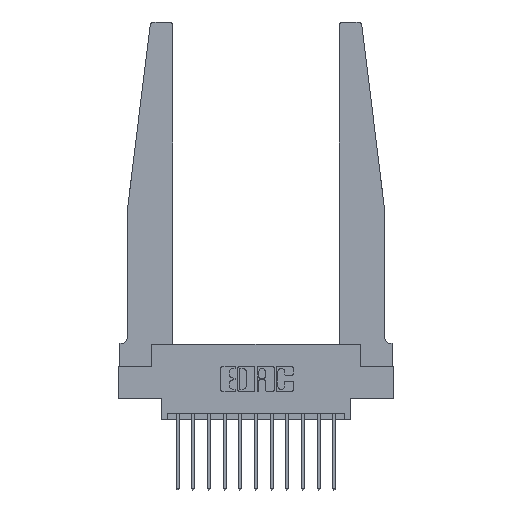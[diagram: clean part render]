
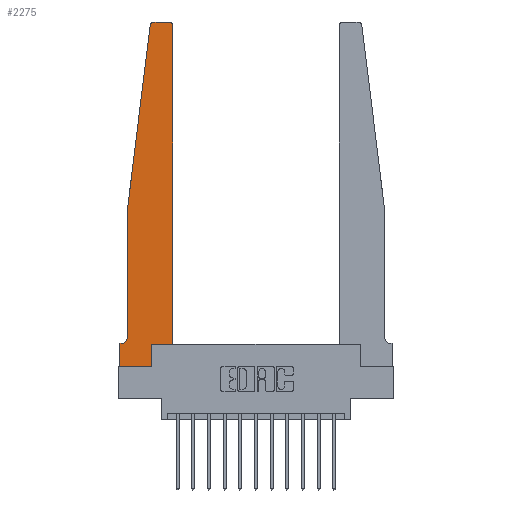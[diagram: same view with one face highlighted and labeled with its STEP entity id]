
A CAD part, top view. The second image highlights one B-rep face of the part: STEP entity #2275.
In plain terms, the highlighted planar face has unit normal (0, 0, 1).
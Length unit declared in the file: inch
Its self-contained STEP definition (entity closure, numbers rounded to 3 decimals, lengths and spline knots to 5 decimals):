
#286 = CARTESIAN_POINT ( 'NONE',  ( 0.425, 0.18, 0.37 ) ) ;
#294 = EDGE_CURVE ( 'NONE', #8847, #5627, #14603, .T. ) ;
#372 = DIRECTION ( 'NONE',  ( 0., -1., 0. ) ) ;
#741 = EDGE_LOOP ( 'NONE', ( #2447, #12523, #12248, #2517, #7901, #7371, #8059, #14027, #2412, #10095, #1513, #2142 ) ) ;
#782 = DIRECTION ( 'NONE',  ( 0., -1., 0. ) ) ;
#792 = CARTESIAN_POINT ( 'NONE',  ( 0.015, 0.1875, 0.37 ) ) ;
#1095 = VERTEX_POINT ( 'NONE', #2716 ) ;
#1129 = CARTESIAN_POINT ( 'NONE',  ( 0.065, 0.1875, 0.37 ) ) ;
#1364 = VERTEX_POINT ( 'NONE', #12464 ) ;
#1419 = CARTESIAN_POINT ( 'NONE',  ( 0.2605, 0.18, 0.37 ) ) ;
#1513 = ORIENTED_EDGE ( 'NONE', *, *, #13581, .T. ) ;
#1672 = CARTESIAN_POINT ( 'NONE',  ( 0.27653, 2.72, 0.37 ) ) ;
#2142 = ORIENTED_EDGE ( 'NONE', *, *, #6327, .T. ) ;
#2221 = DIRECTION ( 'NONE',  ( 0., 0., 1. ) ) ;
#2270 = EDGE_CURVE ( 'NONE', #7335, #9211, #14978, .T. ) ;
#2275 = ADVANCED_FACE ( 'NONE', ( #6229 ), #2309, .T. ) ;
#2309 = PLANE ( 'NONE',  #12874 ) ;
#2319 = VECTOR ( 'NONE', #5821, 39.37008 ) ;
#2369 = EDGE_CURVE ( 'NONE', #9211, #13851, #11251, .T. ) ;
#2412 = ORIENTED_EDGE ( 'NONE', *, *, #15151, .T. ) ;
#2447 = ORIENTED_EDGE ( 'NONE', *, *, #13802, .T. ) ;
#2517 = ORIENTED_EDGE ( 'NONE', *, *, #2270, .T. ) ;
#2583 = LINE ( 'NONE', #10350, #12251 ) ;
#2716 = CARTESIAN_POINT ( 'NONE',  ( 0.27653, 2.75, 0.37 ) ) ;
#2784 = LINE ( 'NONE', #286, #2901 ) ;
#2901 = VECTOR ( 'NONE', #6831, 39.37008 ) ;
#3003 = DIRECTION ( 'NONE',  ( 0., 0., 1. ) ) ;
#3334 = DIRECTION ( 'NONE',  ( 0., 0., -1. ) ) ;
#3445 = VECTOR ( 'NONE', #782, 39.37008 ) ;
#3466 = DIRECTION ( 'NONE',  ( 0., 0., 1. ) ) ;
#3663 = DIRECTION ( 'NONE',  ( -0.122, -0.992, 0. ) ) ;
#4162 = VERTEX_POINT ( 'NONE', #4464 ) ;
#4278 = CARTESIAN_POINT ( 'NONE',  ( 0.2605, 0.18, 0.37 ) ) ;
#4375 = CARTESIAN_POINT ( 'NONE',  ( 0.395, 2.72, 0.37 ) ) ;
#4464 = CARTESIAN_POINT ( 'NONE',  ( 0.2605, 0., 0.37 ) ) ;
#4479 = CARTESIAN_POINT ( 'NONE',  ( 0.425, 0.18, 0.37 ) ) ;
#4486 = AXIS2_PLACEMENT_3D ( 'NONE', #4375, #3003, #5653 ) ;
#4640 = DIRECTION ( 'NONE',  ( -1., 0., 0. ) ) ;
#4787 = LINE ( 'NONE', #11409, #13644 ) ;
#5465 = LINE ( 'NONE', #4278, #9065 ) ;
#5627 = VERTEX_POINT ( 'NONE', #16591 ) ;
#5632 = DIRECTION ( 'NONE',  ( 1., 0., 0. ) ) ;
#5653 = DIRECTION ( 'NONE',  ( 1., 0., 0. ) ) ;
#5821 = DIRECTION ( 'NONE',  ( -1., 0., 0. ) ) ;
#5917 = VECTOR ( 'NONE', #7479, 39.37008 ) ;
#6160 = AXIS2_PLACEMENT_3D ( 'NONE', #13962, #3334, #4640 ) ;
#6229 = FACE_OUTER_BOUND ( 'NONE', #741, .T. ) ;
#6230 = EDGE_CURVE ( 'NONE', #5627, #4162, #2583, .T. ) ;
#6327 = EDGE_CURVE ( 'NONE', #8876, #8344, #7671, .T. ) ;
#6408 = CARTESIAN_POINT ( 'NONE',  ( 0.425, 0.18, 0.37 ) ) ;
#6831 = DIRECTION ( 'NONE',  ( 1., 0., 0. ) ) ;
#7234 = CARTESIAN_POINT ( 'NONE',  ( 0.25, 2.75, 0.37 ) ) ;
#7335 = VERTEX_POINT ( 'NONE', #16352 ) ;
#7371 = ORIENTED_EDGE ( 'NONE', *, *, #10202, .T. ) ;
#7479 = DIRECTION ( 'NONE',  ( -1., 0., 0. ) ) ;
#7504 = LINE ( 'NONE', #6408, #8813 ) ;
#7671 = CIRCLE ( 'NONE', #4486, 0.03 ) ;
#7892 = CARTESIAN_POINT ( 'NONE',  ( 0.395, 2.75, 0.37 ) ) ;
#7901 = ORIENTED_EDGE ( 'NONE', *, *, #2369, .T. ) ;
#7959 = DIRECTION ( 'NONE',  ( 1., 0., 0. ) ) ;
#7999 = EDGE_CURVE ( 'NONE', #1364, #7335, #4787, .T. ) ;
#8059 = ORIENTED_EDGE ( 'NONE', *, *, #294, .T. ) ;
#8125 = EDGE_CURVE ( 'NONE', #1095, #1364, #14757, .T. ) ;
#8344 = VERTEX_POINT ( 'NONE', #7892 ) ;
#8813 = VECTOR ( 'NONE', #15449, 39.37008 ) ;
#8847 = VERTEX_POINT ( 'NONE', #13864 ) ;
#8876 = VERTEX_POINT ( 'NONE', #12436 ) ;
#8888 = CARTESIAN_POINT ( 'NONE',  ( 0.065, 0.2375, 0.37 ) ) ;
#9065 = VECTOR ( 'NONE', #13279, 39.37008 ) ;
#9211 = VERTEX_POINT ( 'NONE', #8888 ) ;
#10095 = ORIENTED_EDGE ( 'NONE', *, *, #10818, .T. ) ;
#10202 = EDGE_CURVE ( 'NONE', #13851, #8847, #15169, .T. ) ;
#10350 = CARTESIAN_POINT ( 'NONE',  ( 0., 0., 0.37 ) ) ;
#10705 = AXIS2_PLACEMENT_3D ( 'NONE', #1672, #3466, #5632 ) ;
#10818 = EDGE_CURVE ( 'NONE', #11677, #14534, #2784, .T. ) ;
#11251 = CIRCLE ( 'NONE', #6160, 0.05 ) ;
#11409 = CARTESIAN_POINT ( 'NONE',  ( 0.065, 1.25, 0.37 ) ) ;
#11677 = VERTEX_POINT ( 'NONE', #1419 ) ;
#12248 = ORIENTED_EDGE ( 'NONE', *, *, #7999, .T. ) ;
#12251 = VECTOR ( 'NONE', #7959, 39.37008 ) ;
#12436 = CARTESIAN_POINT ( 'NONE',  ( 0.425, 2.72, 0.37 ) ) ;
#12464 = CARTESIAN_POINT ( 'NONE',  ( 0.24675, 2.72367, 0.37 ) ) ;
#12523 = ORIENTED_EDGE ( 'NONE', *, *, #8125, .T. ) ;
#12627 = VECTOR ( 'NONE', #372, 39.37008 ) ;
#12874 = AXIS2_PLACEMENT_3D ( 'NONE', #14901, #2221, #13788 ) ;
#13279 = DIRECTION ( 'NONE',  ( 0., 1., 0. ) ) ;
#13581 = EDGE_CURVE ( 'NONE', #14534, #8876, #7504, .T. ) ;
#13644 = VECTOR ( 'NONE', #3663, 39.37008 ) ;
#13788 = DIRECTION ( 'NONE',  ( 1., 0., 0. ) ) ;
#13802 = EDGE_CURVE ( 'NONE', #8344, #1095, #16188, .T. ) ;
#13851 = VERTEX_POINT ( 'NONE', #792 ) ;
#13864 = CARTESIAN_POINT ( 'NONE',  ( 0., 0.1875, 0.37 ) ) ;
#13962 = CARTESIAN_POINT ( 'NONE',  ( 0.015, 0.2375, 0.37 ) ) ;
#14027 = ORIENTED_EDGE ( 'NONE', *, *, #6230, .T. ) ;
#14534 = VERTEX_POINT ( 'NONE', #4479 ) ;
#14603 = LINE ( 'NONE', #15884, #12627 ) ;
#14757 = CIRCLE ( 'NONE', #10705, 0.03 ) ;
#14901 = CARTESIAN_POINT ( 'NONE',  ( 0., 0.1875, 0.37 ) ) ;
#14978 = LINE ( 'NONE', #16415, #3445 ) ;
#15151 = EDGE_CURVE ( 'NONE', #4162, #11677, #5465, .T. ) ;
#15169 = LINE ( 'NONE', #1129, #5917 ) ;
#15449 = DIRECTION ( 'NONE',  ( 0., 1., 0. ) ) ;
#15884 = CARTESIAN_POINT ( 'NONE',  ( 0., 0., 0.37 ) ) ;
#16188 = LINE ( 'NONE', #7234, #2319 ) ;
#16352 = CARTESIAN_POINT ( 'NONE',  ( 0.065, 1.25, 0.37 ) ) ;
#16415 = CARTESIAN_POINT ( 'NONE',  ( 0.065, 1.25, 0.37 ) ) ;
#16591 = CARTESIAN_POINT ( 'NONE',  ( 0., 0., 0.37 ) ) ;
